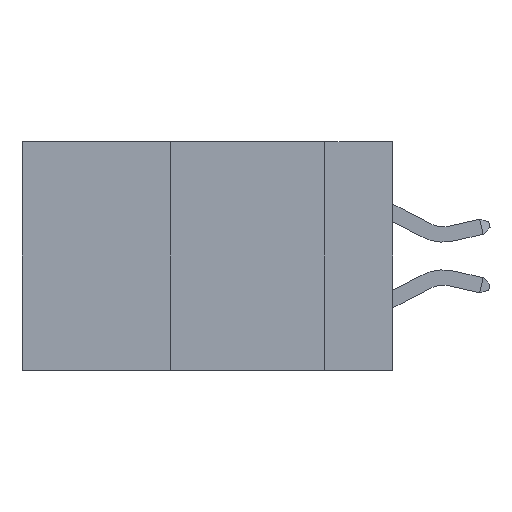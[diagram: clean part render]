
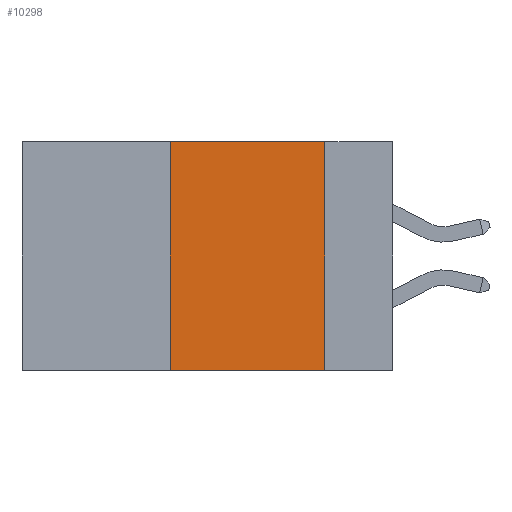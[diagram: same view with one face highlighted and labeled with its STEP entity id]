
A CAD part, left-side view. The second image highlights one B-rep face of the part: STEP entity #10298.
In plain terms, the highlighted planar face has unit normal (-1, 0, 0).
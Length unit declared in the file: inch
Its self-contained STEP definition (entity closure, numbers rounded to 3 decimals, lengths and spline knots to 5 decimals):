
#94 = EDGE_CURVE ( 'NONE', #9058, #1449, #3021, .T. ) ;
#1066 = CARTESIAN_POINT ( 'NONE',  ( 0., 0.6, 0. ) ) ;
#1102 = DIRECTION ( 'NONE',  ( 0., 0., -1. ) ) ;
#1125 = VERTEX_POINT ( 'NONE', #5433 ) ;
#1155 = AXIS2_PLACEMENT_3D ( 'NONE', #1066, #6033, #1102 ) ;
#1389 = VECTOR ( 'NONE', #5628, 39.37008 ) ;
#1449 = VERTEX_POINT ( 'NONE', #4847 ) ;
#1705 = DIRECTION ( 'NONE',  ( 0., -1., 0. ) ) ;
#2214 = EDGE_CURVE ( 'NONE', #3709, #1125, #3725, .T. ) ;
#2650 = VECTOR ( 'NONE', #7525, 39.37008 ) ;
#2766 = CARTESIAN_POINT ( 'NONE',  ( 0., 0.11, 0. ) ) ;
#3021 = LINE ( 'NONE', #7548, #9140 ) ;
#3709 = VERTEX_POINT ( 'NONE', #9641 ) ;
#3725 = LINE ( 'NONE', #8541, #7208 ) ;
#3919 = ORIENTED_EDGE ( 'NONE', *, *, #10024, .F. ) ;
#4638 = FACE_OUTER_BOUND ( 'NONE', #6986, .T. ) ;
#4847 = CARTESIAN_POINT ( 'NONE',  ( 0., 0.11, 0. ) ) ;
#5433 = CARTESIAN_POINT ( 'NONE',  ( 0., 0.11, -0.37 ) ) ;
#5628 = DIRECTION ( 'NONE',  ( 0., 0., 1. ) ) ;
#5926 = ORIENTED_EDGE ( 'NONE', *, *, #9608, .F. ) ;
#6033 = DIRECTION ( 'NONE',  ( 1., 0., 0. ) ) ;
#6165 = ORIENTED_EDGE ( 'NONE', *, *, #2214, .T. ) ;
#6986 = EDGE_LOOP ( 'NONE', ( #5926, #9049, #3919, #6165 ) ) ;
#7208 = VECTOR ( 'NONE', #8460, 39.37008 ) ;
#7525 = DIRECTION ( 'NONE',  ( 0., 0., -1. ) ) ;
#7548 = CARTESIAN_POINT ( 'NONE',  ( 0., 0.6, 0. ) ) ;
#8460 = DIRECTION ( 'NONE',  ( 0., -1., 0. ) ) ;
#8541 = CARTESIAN_POINT ( 'NONE',  ( 0., 0.6, -0.37 ) ) ;
#8772 = CARTESIAN_POINT ( 'NONE',  ( 0., 0.36, 0. ) ) ;
#9023 = LINE ( 'NONE', #2766, #2650 ) ;
#9049 = ORIENTED_EDGE ( 'NONE', *, *, #94, .F. ) ;
#9058 = VERTEX_POINT ( 'NONE', #9251 ) ;
#9140 = VECTOR ( 'NONE', #1705, 39.37008 ) ;
#9251 = CARTESIAN_POINT ( 'NONE',  ( 0., 0.36, 0. ) ) ;
#9608 = EDGE_CURVE ( 'NONE', #1449, #1125, #9023, .T. ) ;
#9641 = CARTESIAN_POINT ( 'NONE',  ( 0., 0.36, -0.37 ) ) ;
#10004 = PLANE ( 'NONE',  #1155 ) ;
#10006 = LINE ( 'NONE', #8772, #1389 ) ;
#10024 = EDGE_CURVE ( 'NONE', #3709, #9058, #10006, .T. ) ;
#10298 = ADVANCED_FACE ( 'NONE', ( #4638 ), #10004, .F. ) ;
